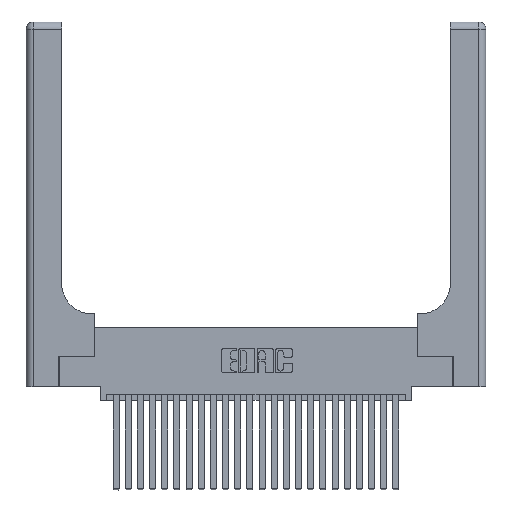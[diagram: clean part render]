
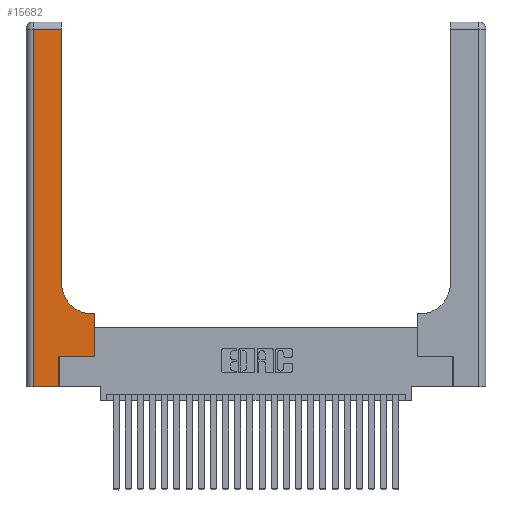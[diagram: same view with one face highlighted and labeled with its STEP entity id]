
A CAD part, top view. The second image highlights one B-rep face of the part: STEP entity #15682.
In plain terms, the highlighted planar face has unit normal (0, 0, 1).
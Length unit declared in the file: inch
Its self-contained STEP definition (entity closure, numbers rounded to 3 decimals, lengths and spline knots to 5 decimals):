
#61 = VECTOR ( 'NONE', #3644, 39.37008 ) ;
#403 = PLANE ( 'NONE',  #14028 ) ;
#433 = VERTEX_POINT ( 'NONE', #5666 ) ;
#502 = LINE ( 'NONE', #19309, #18707 ) ;
#756 = VERTEX_POINT ( 'NONE', #26386 ) ;
#949 = DIRECTION ( 'NONE',  ( 1., 0., 0. ) ) ;
#1075 = DIRECTION ( 'NONE',  ( -1., 0., 0. ) ) ;
#3356 = EDGE_CURVE ( 'NONE', #433, #12272, #11876, .T. ) ;
#3644 = DIRECTION ( 'NONE',  ( 0., 1., 0. ) ) ;
#3825 = ORIENTED_EDGE ( 'NONE', *, *, #3356, .T. ) ;
#4204 = CARTESIAN_POINT ( 'NONE',  ( 0.5415, 0.85, 0.37 ) ) ;
#5191 = EDGE_CURVE ( 'NONE', #12272, #20864, #13915, .T. ) ;
#5212 = ORIENTED_EDGE ( 'NONE', *, *, #22110, .T. ) ;
#5666 = CARTESIAN_POINT ( 'NONE',  ( 0.269, 0., 0.37 ) ) ;
#5780 = LINE ( 'NONE', #7573, #24235 ) ;
#6411 = VERTEX_POINT ( 'NONE', #17995 ) ;
#6583 = DIRECTION ( 'NONE',  ( -1., 0., 0. ) ) ;
#7015 = VERTEX_POINT ( 'NONE', #14796 ) ;
#7156 = EDGE_CURVE ( 'NONE', #22385, #6411, #21509, .T. ) ;
#7573 = CARTESIAN_POINT ( 'NONE',  ( 0.5585, 0.25, 0.37 ) ) ;
#8322 = EDGE_CURVE ( 'NONE', #756, #17477, #15437, .T. ) ;
#8573 = CARTESIAN_POINT ( 'NONE',  ( 0.269, 0., 0.37 ) ) ;
#10266 = FACE_OUTER_BOUND ( 'NONE', #19771, .T. ) ;
#10345 = CARTESIAN_POINT ( 'NONE',  ( 0.5415, 0.6, 0.37 ) ) ;
#10472 = ORIENTED_EDGE ( 'NONE', *, *, #7156, .T. ) ;
#10495 = CARTESIAN_POINT ( 'NONE',  ( 0.5585, 0.25, 0.37 ) ) ;
#10549 = ORIENTED_EDGE ( 'NONE', *, *, #5191, .T. ) ;
#10564 = CARTESIAN_POINT ( 'NONE',  ( 0.06, 3., 0.37 ) ) ;
#11001 = LINE ( 'NONE', #20690, #22781 ) ;
#11667 = EDGE_CURVE ( 'NONE', #20864, #12071, #5780, .T. ) ;
#11876 = LINE ( 'NONE', #8573, #61 ) ;
#12071 = VERTEX_POINT ( 'NONE', #19063 ) ;
#12139 = DIRECTION ( 'NONE',  ( 0., -1., 0. ) ) ;
#12145 = DIRECTION ( 'NONE',  ( 0., 1., 0. ) ) ;
#12272 = VERTEX_POINT ( 'NONE', #25918 ) ;
#12490 = DIRECTION ( 'NONE',  ( 1., 0., 0. ) ) ;
#12575 = CARTESIAN_POINT ( 'NONE',  ( 0., 2.94, 0.37 ) ) ;
#13399 = LINE ( 'NONE', #16122, #22945 ) ;
#13894 = LINE ( 'NONE', #12575, #14223 ) ;
#13915 = LINE ( 'NONE', #25121, #25372 ) ;
#14028 = AXIS2_PLACEMENT_3D ( 'NONE', #18625, #16875, #6583 ) ;
#14223 = VECTOR ( 'NONE', #20483, 39.37008 ) ;
#14796 = CARTESIAN_POINT ( 'NONE',  ( 0.2915, 2.94, 0.37 ) ) ;
#15437 = LINE ( 'NONE', #10564, #23688 ) ;
#15670 = ORIENTED_EDGE ( 'NONE', *, *, #8322, .T. ) ;
#15682 = ADVANCED_FACE ( 'NONE', ( #10266 ), #403, .F. ) ;
#16122 = CARTESIAN_POINT ( 'NONE',  ( 0.2915, 3., 0.37 ) ) ;
#16535 = DIRECTION ( 'NONE',  ( 0., 0., -1. ) ) ;
#16833 = DIRECTION ( 'NONE',  ( 1., 0., 0. ) ) ;
#16867 = ORIENTED_EDGE ( 'NONE', *, *, #11667, .T. ) ;
#16875 = DIRECTION ( 'NONE',  ( 0., 0., -1. ) ) ;
#17060 = ORIENTED_EDGE ( 'NONE', *, *, #18598, .T. ) ;
#17166 = EDGE_CURVE ( 'NONE', #6411, #7015, #13399, .T. ) ;
#17477 = VERTEX_POINT ( 'NONE', #22001 ) ;
#17995 = CARTESIAN_POINT ( 'NONE',  ( 0.2915, 0.85, 0.37 ) ) ;
#18598 = EDGE_CURVE ( 'NONE', #12071, #22385, #502, .T. ) ;
#18625 = CARTESIAN_POINT ( 'NONE',  ( 0., 3., 0.37 ) ) ;
#18707 = VECTOR ( 'NONE', #1075, 39.37008 ) ;
#19063 = CARTESIAN_POINT ( 'NONE',  ( 0.5585, 0.6, 0.37 ) ) ;
#19225 = AXIS2_PLACEMENT_3D ( 'NONE', #4204, #16535, #12490 ) ;
#19309 = CARTESIAN_POINT ( 'NONE',  ( 0.2915, 0.6, 0.37 ) ) ;
#19482 = EDGE_CURVE ( 'NONE', #17477, #433, #11001, .T. ) ;
#19771 = EDGE_LOOP ( 'NONE', ( #20951, #5212, #15670, #20106, #3825, #10549, #16867, #17060, #10472 ) ) ;
#20106 = ORIENTED_EDGE ( 'NONE', *, *, #19482, .T. ) ;
#20483 = DIRECTION ( 'NONE',  ( -1., 0., 0. ) ) ;
#20690 = CARTESIAN_POINT ( 'NONE',  ( 0., 0., 0.37 ) ) ;
#20864 = VERTEX_POINT ( 'NONE', #10495 ) ;
#20951 = ORIENTED_EDGE ( 'NONE', *, *, #17166, .T. ) ;
#21509 = CIRCLE ( 'NONE', #19225, 0.25 ) ;
#21784 = DIRECTION ( 'NONE',  ( 0., 1., 0. ) ) ;
#22001 = CARTESIAN_POINT ( 'NONE',  ( 0.06, 0., 0.37 ) ) ;
#22110 = EDGE_CURVE ( 'NONE', #7015, #756, #13894, .T. ) ;
#22385 = VERTEX_POINT ( 'NONE', #10345 ) ;
#22781 = VECTOR ( 'NONE', #16833, 39.37008 ) ;
#22945 = VECTOR ( 'NONE', #12145, 39.37008 ) ;
#23688 = VECTOR ( 'NONE', #12139, 39.37008 ) ;
#24235 = VECTOR ( 'NONE', #21784, 39.37008 ) ;
#25121 = CARTESIAN_POINT ( 'NONE',  ( 0.269, 0.25, 0.37 ) ) ;
#25372 = VECTOR ( 'NONE', #949, 39.37008 ) ;
#25918 = CARTESIAN_POINT ( 'NONE',  ( 0.269, 0.25, 0.37 ) ) ;
#26386 = CARTESIAN_POINT ( 'NONE',  ( 0.06, 2.94, 0.37 ) ) ;
